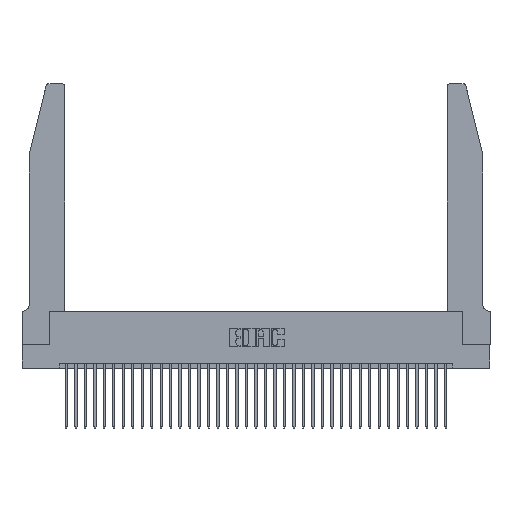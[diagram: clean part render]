
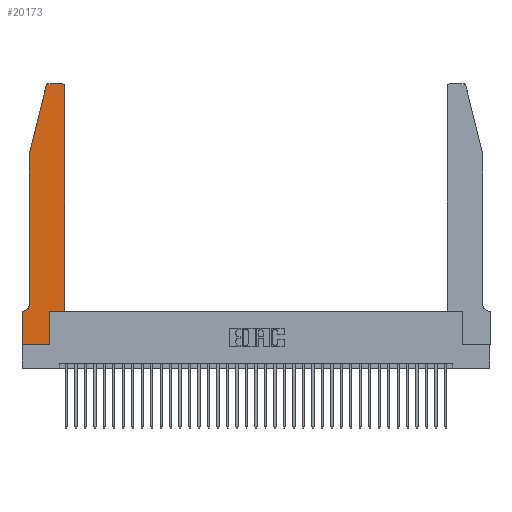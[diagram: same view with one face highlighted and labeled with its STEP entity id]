
A CAD part, top view. The second image highlights one B-rep face of the part: STEP entity #20173.
In plain terms, the highlighted planar face has unit normal (0, 0, 1).
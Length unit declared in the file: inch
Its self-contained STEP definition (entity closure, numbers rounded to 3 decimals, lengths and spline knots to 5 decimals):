
#421 = ORIENTED_EDGE ( 'NONE', *, *, #35796, .T. ) ;
#562 = VERTEX_POINT ( 'NONE', #28622 ) ;
#666 = VECTOR ( 'NONE', #9497, 39.37008 ) ;
#694 = CARTESIAN_POINT ( 'NONE',  ( 0.284, 2.72, 0.37 ) ) ;
#695 = LINE ( 'NONE', #11904, #13651 ) ;
#1357 = VECTOR ( 'NONE', #32507, 39.37008 ) ;
#1738 = EDGE_CURVE ( 'NONE', #33949, #20953, #18231, .T. ) ;
#2305 = CARTESIAN_POINT ( 'NONE',  ( 0., 0.35, 0.37 ) ) ;
#3653 = CARTESIAN_POINT ( 'NONE',  ( 0.4505, 0.35, 0.37 ) ) ;
#3705 = CIRCLE ( 'NONE', #6801, 0.03 ) ;
#4740 = VERTEX_POINT ( 'NONE', #18142 ) ;
#5033 = VECTOR ( 'NONE', #24555, 39.37008 ) ;
#5156 = CARTESIAN_POINT ( 'NONE',  ( 0., 0., 0.37 ) ) ;
#5284 = DIRECTION ( 'NONE',  ( 0., 0., 1. ) ) ;
#5876 = CARTESIAN_POINT ( 'NONE',  ( 0.284, 2.75, 0.37 ) ) ;
#6026 = LINE ( 'NONE', #20310, #30272 ) ;
#6439 = EDGE_CURVE ( 'NONE', #9073, #8053, #18661, .T. ) ;
#6534 = VERTEX_POINT ( 'NONE', #9546 ) ;
#6641 = ORIENTED_EDGE ( 'NONE', *, *, #20673, .T. ) ;
#6801 = AXIS2_PLACEMENT_3D ( 'NONE', #694, #23303, #20046 ) ;
#6968 = DIRECTION ( 'NONE',  ( 0., -1., 0. ) ) ;
#7895 = VECTOR ( 'NONE', #11706, 39.37008 ) ;
#8053 = VERTEX_POINT ( 'NONE', #36157 ) ;
#8516 = DIRECTION ( 'NONE',  ( 1., 0., 0. ) ) ;
#8756 = DIRECTION ( 'NONE',  ( -1., 0., 0. ) ) ;
#8786 = DIRECTION ( 'NONE',  ( 1., 0., 0. ) ) ;
#8938 = LINE ( 'NONE', #18217, #1357 ) ;
#9073 = VERTEX_POINT ( 'NONE', #3653 ) ;
#9497 = DIRECTION ( 'NONE',  ( 0., 1., 0. ) ) ;
#9546 = CARTESIAN_POINT ( 'NONE',  ( 0., 0.35, 0.37 ) ) ;
#10360 = DIRECTION ( 'NONE',  ( 0., 0., -1. ) ) ;
#11084 = EDGE_CURVE ( 'NONE', #4740, #26765, #27896, .T. ) ;
#11706 = DIRECTION ( 'NONE',  ( 0., 1., 0. ) ) ;
#11904 = CARTESIAN_POINT ( 'NONE',  ( 0., 0., 0.37 ) ) ;
#12337 = ORIENTED_EDGE ( 'NONE', *, *, #33640, .T. ) ;
#12494 = VERTEX_POINT ( 'NONE', #21850 ) ;
#12885 = DIRECTION ( 'NONE',  ( -1., 0., 0. ) ) ;
#13651 = VECTOR ( 'NONE', #17653, 39.37008 ) ;
#13909 = ORIENTED_EDGE ( 'NONE', *, *, #11084, .T. ) ;
#13920 = PLANE ( 'NONE',  #24101 ) ;
#15979 = ORIENTED_EDGE ( 'NONE', *, *, #17739, .T. ) ;
#16807 = ORIENTED_EDGE ( 'NONE', *, *, #33979, .T. ) ;
#16943 = CARTESIAN_POINT ( 'NONE',  ( 0.4205, 2.72, 0.37 ) ) ;
#17653 = DIRECTION ( 'NONE',  ( 0., -1., 0. ) ) ;
#17739 = EDGE_CURVE ( 'NONE', #28689, #6534, #6026, .T. ) ;
#17762 = EDGE_CURVE ( 'NONE', #6534, #562, #695, .T. ) ;
#18142 = CARTESIAN_POINT ( 'NONE',  ( 0.4205, 2.75, 0.37 ) ) ;
#18217 = CARTESIAN_POINT ( 'NONE',  ( 0.4505, 0.35, 0.37 ) ) ;
#18231 = LINE ( 'NONE', #30275, #20483 ) ;
#18661 = LINE ( 'NONE', #26106, #7895 ) ;
#18866 = VERTEX_POINT ( 'NONE', #19385 ) ;
#19385 = CARTESIAN_POINT ( 'NONE',  ( 0.2865, 0., 0.37 ) ) ;
#20046 = DIRECTION ( 'NONE',  ( 1., 0., 0. ) ) ;
#20173 = ADVANCED_FACE ( 'NONE', ( #32102 ), #13920, .T. ) ;
#20310 = CARTESIAN_POINT ( 'NONE',  ( 0.0755, 0.35, 0.37 ) ) ;
#20418 = EDGE_CURVE ( 'NONE', #26765, #36249, #3705, .T. ) ;
#20483 = VECTOR ( 'NONE', #6968, 39.37008 ) ;
#20673 = EDGE_CURVE ( 'NONE', #20953, #28689, #35503, .T. ) ;
#20953 = VERTEX_POINT ( 'NONE', #25640 ) ;
#21529 = CARTESIAN_POINT ( 'NONE',  ( 0.0055, 0.42, 0.37 ) ) ;
#21761 = AXIS2_PLACEMENT_3D ( 'NONE', #16943, #28326, #8786 ) ;
#21850 = CARTESIAN_POINT ( 'NONE',  ( 0.2865, 0.35, 0.37 ) ) ;
#22249 = ORIENTED_EDGE ( 'NONE', *, *, #6439, .T. ) ;
#22295 = EDGE_CURVE ( 'NONE', #12494, #9073, #8938, .T. ) ;
#22306 = CIRCLE ( 'NONE', #21761, 0.03 ) ;
#22912 = CARTESIAN_POINT ( 'NONE',  ( 0.25487, 2.72718, 0.37 ) ) ;
#23160 = LINE ( 'NONE', #5156, #25850 ) ;
#23303 = DIRECTION ( 'NONE',  ( 0., 0., 1. ) ) ;
#23829 = ORIENTED_EDGE ( 'NONE', *, *, #20418, .T. ) ;
#23875 = LINE ( 'NONE', #23929, #24760 ) ;
#23929 = CARTESIAN_POINT ( 'NONE',  ( 0.0755, 2., 0.37 ) ) ;
#24101 = AXIS2_PLACEMENT_3D ( 'NONE', #2305, #5284, #8516 ) ;
#24497 = ORIENTED_EDGE ( 'NONE', *, *, #24528, .T. ) ;
#24528 = EDGE_CURVE ( 'NONE', #36249, #33949, #23875, .T. ) ;
#24555 = DIRECTION ( 'NONE',  ( -1., 0., 0. ) ) ;
#24760 = VECTOR ( 'NONE', #32918, 39.37008 ) ;
#25640 = CARTESIAN_POINT ( 'NONE',  ( 0.0755, 0.42, 0.37 ) ) ;
#25827 = ORIENTED_EDGE ( 'NONE', *, *, #1738, .T. ) ;
#25850 = VECTOR ( 'NONE', #33710, 39.37008 ) ;
#26106 = CARTESIAN_POINT ( 'NONE',  ( 0.4505, 0.35, 0.37 ) ) ;
#26765 = VERTEX_POINT ( 'NONE', #5876 ) ;
#27896 = LINE ( 'NONE', #33060, #5033 ) ;
#27955 = CARTESIAN_POINT ( 'NONE',  ( 0.0755, 2., 0.37 ) ) ;
#28326 = DIRECTION ( 'NONE',  ( 0., 0., 1. ) ) ;
#28622 = CARTESIAN_POINT ( 'NONE',  ( 0., 0., 0.37 ) ) ;
#28689 = VERTEX_POINT ( 'NONE', #31540 ) ;
#30272 = VECTOR ( 'NONE', #8756, 39.37008 ) ;
#30275 = CARTESIAN_POINT ( 'NONE',  ( 0.0755, 2., 0.37 ) ) ;
#30475 = EDGE_LOOP ( 'NONE', ( #13909, #23829, #24497, #25827, #6641, #15979, #36227, #16807, #421, #32956, #22249, #12337 ) ) ;
#31540 = CARTESIAN_POINT ( 'NONE',  ( 0.0055, 0.35, 0.37 ) ) ;
#32102 = FACE_OUTER_BOUND ( 'NONE', #30475, .T. ) ;
#32491 = AXIS2_PLACEMENT_3D ( 'NONE', #21529, #10360, #12885 ) ;
#32507 = DIRECTION ( 'NONE',  ( 1., 0., 0. ) ) ;
#32918 = DIRECTION ( 'NONE',  ( -0.239, -0.971, 0. ) ) ;
#32956 = ORIENTED_EDGE ( 'NONE', *, *, #22295, .T. ) ;
#33060 = CARTESIAN_POINT ( 'NONE',  ( 0.2605, 2.75, 0.37 ) ) ;
#33360 = LINE ( 'NONE', #35184, #666 ) ;
#33640 = EDGE_CURVE ( 'NONE', #8053, #4740, #22306, .T. ) ;
#33710 = DIRECTION ( 'NONE',  ( 1., 0., 0. ) ) ;
#33949 = VERTEX_POINT ( 'NONE', #27955 ) ;
#33979 = EDGE_CURVE ( 'NONE', #562, #18866, #23160, .T. ) ;
#35184 = CARTESIAN_POINT ( 'NONE',  ( 0.2865, 0.35, 0.37 ) ) ;
#35503 = CIRCLE ( 'NONE', #32491, 0.07 ) ;
#35796 = EDGE_CURVE ( 'NONE', #18866, #12494, #33360, .T. ) ;
#36157 = CARTESIAN_POINT ( 'NONE',  ( 0.4505, 2.72, 0.37 ) ) ;
#36227 = ORIENTED_EDGE ( 'NONE', *, *, #17762, .T. ) ;
#36249 = VERTEX_POINT ( 'NONE', #22912 ) ;
